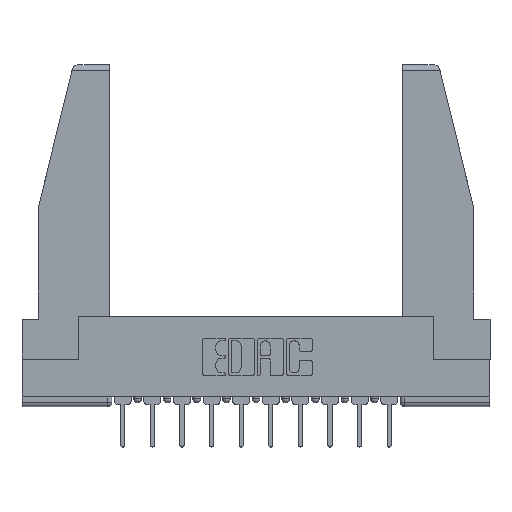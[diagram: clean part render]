
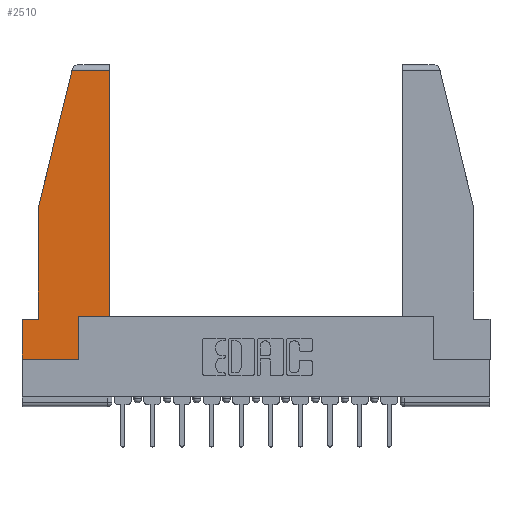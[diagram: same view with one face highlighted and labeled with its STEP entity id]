
A CAD part, top view. The second image highlights one B-rep face of the part: STEP entity #2510.
In plain terms, the highlighted planar face has unit normal (0, 0, 1).
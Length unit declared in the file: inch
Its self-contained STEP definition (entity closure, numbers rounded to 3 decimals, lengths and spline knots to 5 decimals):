
#187 = CARTESIAN_POINT ( 'NONE',  ( 0., 0.21, 0. ) ) ;
#434 = AXIS2_PLACEMENT_3D ( 'NONE', #4231, #2988, #6354 ) ;
#481 = VECTOR ( 'NONE', #5980, 39.37008 ) ;
#517 = CARTESIAN_POINT ( 'NONE',  ( 0.2636, 1.52, 0. ) ) ;
#528 = VERTEX_POINT ( 'NONE', #13907 ) ;
#773 = EDGE_CURVE ( 'NONE', #528, #8259, #13555, .T. ) ;
#810 = ORIENTED_EDGE ( 'NONE', *, *, #2971, .T. ) ;
#1370 = DIRECTION ( 'NONE',  ( 0., 1., 0. ) ) ;
#1525 = CARTESIAN_POINT ( 'NONE',  ( 0., 0., 0. ) ) ;
#2510 = ADVANCED_FACE ( 'NONE', ( #3828 ), #14711, .T. ) ;
#2573 = LINE ( 'NONE', #5219, #8637 ) ;
#2669 = LINE ( 'NONE', #11216, #5067 ) ;
#2816 = EDGE_CURVE ( 'NONE', #8259, #4744, #13573, .T. ) ;
#2971 = EDGE_CURVE ( 'NONE', #14635, #6776, #11365, .T. ) ;
#2988 = DIRECTION ( 'NONE',  ( 0., 0., 1. ) ) ;
#3360 = ORIENTED_EDGE ( 'NONE', *, *, #15185, .T. ) ;
#3585 = VECTOR ( 'NONE', #12215, 39.37008 ) ;
#3631 = VECTOR ( 'NONE', #15070, 39.37008 ) ;
#3828 = FACE_OUTER_BOUND ( 'NONE', #12732, .T. ) ;
#3918 = LINE ( 'NONE', #6929, #3937 ) ;
#3931 = VECTOR ( 'NONE', #1370, 39.37008 ) ;
#3937 = VECTOR ( 'NONE', #15188, 39.37008 ) ;
#4094 = ORIENTED_EDGE ( 'NONE', *, *, #2816, .T. ) ;
#4222 = EDGE_CURVE ( 'NONE', #6776, #12901, #5961, .T. ) ;
#4231 = CARTESIAN_POINT ( 'NONE',  ( 0., 0., 0. ) ) ;
#4431 = EDGE_CURVE ( 'NONE', #12211, #10301, #2669, .T. ) ;
#4525 = VECTOR ( 'NONE', #8285, 39.37008 ) ;
#4744 = VERTEX_POINT ( 'NONE', #1525 ) ;
#4762 = EDGE_CURVE ( 'NONE', #8653, #12211, #13151, .T. ) ;
#5067 = VECTOR ( 'NONE', #6575, 39.37008 ) ;
#5219 = CARTESIAN_POINT ( 'NONE',  ( 0.086, 0.8, 0. ) ) ;
#5543 = EDGE_CURVE ( 'NONE', #10301, #14635, #3918, .T. ) ;
#5772 = LINE ( 'NONE', #6437, #3585 ) ;
#5959 = ORIENTED_EDGE ( 'NONE', *, *, #4431, .T. ) ;
#5961 = LINE ( 'NONE', #14165, #4525 ) ;
#5980 = DIRECTION ( 'NONE',  ( -1., 0., 0. ) ) ;
#6354 = DIRECTION ( 'NONE',  ( 1., 0., 0. ) ) ;
#6437 = CARTESIAN_POINT ( 'NONE',  ( 0., 0., 0. ) ) ;
#6575 = DIRECTION ( 'NONE',  ( 1., 0., 0. ) ) ;
#6581 = DIRECTION ( 'NONE',  ( 0., -1., 0. ) ) ;
#6776 = VERTEX_POINT ( 'NONE', #517 ) ;
#6796 = CARTESIAN_POINT ( 'NONE',  ( 0.297, 0., 0. ) ) ;
#6929 = CARTESIAN_POINT ( 'NONE',  ( 0.461, 0.223, 0. ) ) ;
#7218 = CARTESIAN_POINT ( 'NONE',  ( 0.297, 0., 0. ) ) ;
#7658 = VECTOR ( 'NONE', #10799, 39.37008 ) ;
#7687 = CARTESIAN_POINT ( 'NONE',  ( 0.297, 0.223, 0. ) ) ;
#7742 = ORIENTED_EDGE ( 'NONE', *, *, #5543, .T. ) ;
#7914 = ORIENTED_EDGE ( 'NONE', *, *, #8408, .T. ) ;
#8202 = CARTESIAN_POINT ( 'NONE',  ( 0., 0.21, 0. ) ) ;
#8259 = VERTEX_POINT ( 'NONE', #9534 ) ;
#8285 = DIRECTION ( 'NONE',  ( -0.239, -0.971, 0. ) ) ;
#8408 = EDGE_CURVE ( 'NONE', #4744, #8653, #5772, .T. ) ;
#8637 = VECTOR ( 'NONE', #6581, 39.37008 ) ;
#8653 = VERTEX_POINT ( 'NONE', #6796 ) ;
#8864 = CARTESIAN_POINT ( 'NONE',  ( 0.086, 0.8, 0. ) ) ;
#9534 = CARTESIAN_POINT ( 'NONE',  ( 0., 0.21, 0. ) ) ;
#9862 = CARTESIAN_POINT ( 'NONE',  ( 0.461, 1.52, 0. ) ) ;
#10301 = VERTEX_POINT ( 'NONE', #12173 ) ;
#10799 = DIRECTION ( 'NONE',  ( -1., 0., 0. ) ) ;
#10840 = ORIENTED_EDGE ( 'NONE', *, *, #4222, .T. ) ;
#11216 = CARTESIAN_POINT ( 'NONE',  ( 0.297, 0.223, 0. ) ) ;
#11365 = LINE ( 'NONE', #13048, #481 ) ;
#12173 = CARTESIAN_POINT ( 'NONE',  ( 0.461, 0.223, 0. ) ) ;
#12211 = VERTEX_POINT ( 'NONE', #7687 ) ;
#12215 = DIRECTION ( 'NONE',  ( 1., 0., 0. ) ) ;
#12732 = EDGE_LOOP ( 'NONE', ( #7742, #810, #10840, #3360, #13092, #4094, #7914, #15271, #5959 ) ) ;
#12901 = VERTEX_POINT ( 'NONE', #8864 ) ;
#13048 = CARTESIAN_POINT ( 'NONE',  ( 0., 1.52, 0. ) ) ;
#13092 = ORIENTED_EDGE ( 'NONE', *, *, #773, .T. ) ;
#13151 = LINE ( 'NONE', #7218, #3931 ) ;
#13555 = LINE ( 'NONE', #187, #7658 ) ;
#13573 = LINE ( 'NONE', #8202, #3631 ) ;
#13907 = CARTESIAN_POINT ( 'NONE',  ( 0.086, 0.21, 0. ) ) ;
#14165 = CARTESIAN_POINT ( 'NONE',  ( 0.271, 1.55, 0. ) ) ;
#14635 = VERTEX_POINT ( 'NONE', #9862 ) ;
#14711 = PLANE ( 'NONE',  #434 ) ;
#15070 = DIRECTION ( 'NONE',  ( 0., -1., 0. ) ) ;
#15185 = EDGE_CURVE ( 'NONE', #12901, #528, #2573, .T. ) ;
#15188 = DIRECTION ( 'NONE',  ( 0., 1., 0. ) ) ;
#15271 = ORIENTED_EDGE ( 'NONE', *, *, #4762, .T. ) ;
